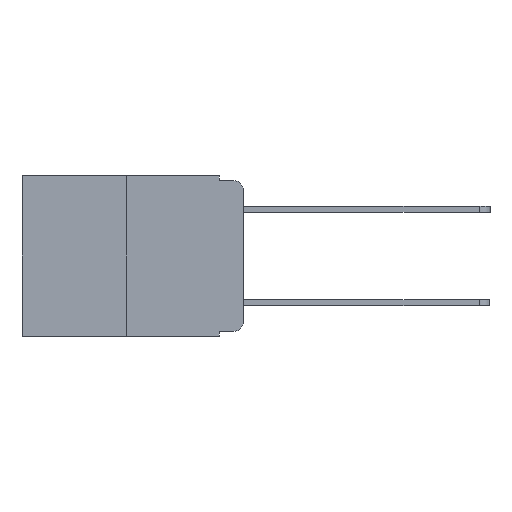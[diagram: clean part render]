
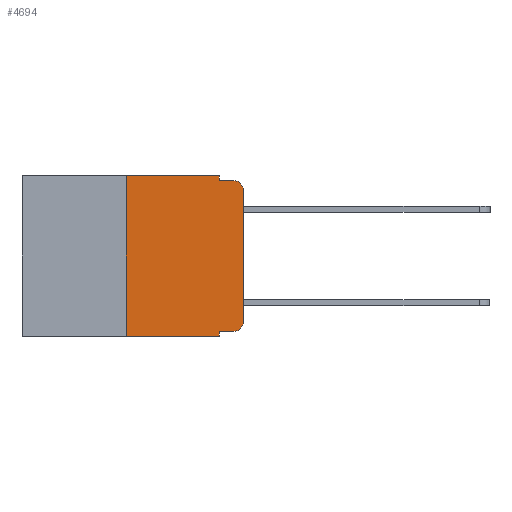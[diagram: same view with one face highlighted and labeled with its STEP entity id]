
A CAD part, left-side view. The second image highlights one B-rep face of the part: STEP entity #4694.
In plain terms, the highlighted planar face has unit normal (-1, 0, 0).
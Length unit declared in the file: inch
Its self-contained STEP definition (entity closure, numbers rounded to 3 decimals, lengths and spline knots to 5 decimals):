
#53 = VERTEX_POINT ( 'NONE', #17439 ) ;
#73 = LINE ( 'NONE', #3308, #14886 ) ;
#321 = VERTEX_POINT ( 'NONE', #8775 ) ;
#516 = VERTEX_POINT ( 'NONE', #12780 ) ;
#943 = CARTESIAN_POINT ( 'NONE',  ( 0., 0.02, -0.01 ) ) ;
#1079 = EDGE_CURVE ( 'NONE', #13276, #7350, #13973, .T. ) ;
#1760 = CARTESIAN_POINT ( 'NONE',  ( 0., 0.051, -0.333 ) ) ;
#1866 = VECTOR ( 'NONE', #15517, 39.37008 ) ;
#1923 = CARTESIAN_POINT ( 'NONE',  ( 0., 0.051, -0.01 ) ) ;
#2080 = EDGE_CURVE ( 'NONE', #9093, #53, #17337, .T. ) ;
#3308 = CARTESIAN_POINT ( 'NONE',  ( 0., 0.25, 0. ) ) ;
#3718 = VERTEX_POINT ( 'NONE', #943 ) ;
#3802 = VERTEX_POINT ( 'NONE', #11921 ) ;
#4694 = ADVANCED_FACE ( 'NONE', ( #8279 ), #8007, .F. ) ;
#4800 = EDGE_CURVE ( 'NONE', #3802, #321, #13124, .T. ) ;
#4819 = CARTESIAN_POINT ( 'NONE',  ( 0., 0.051, -0.333 ) ) ;
#4912 = VECTOR ( 'NONE', #18593, 39.37008 ) ;
#4969 = LINE ( 'NONE', #14575, #16102 ) ;
#5152 = EDGE_CURVE ( 'NONE', #516, #3718, #18924, .T. ) ;
#5221 = VECTOR ( 'NONE', #10815, 39.37008 ) ;
#5332 = ORIENTED_EDGE ( 'NONE', *, *, #12474, .T. ) ;
#5348 = DIRECTION ( 'NONE',  ( 0., -1., 0. ) ) ;
#6145 = EDGE_LOOP ( 'NONE', ( #15841, #15179, #15151, #14642, #14334, #14672, #7947, #7739, #6609, #5332 ) ) ;
#6278 = DIRECTION ( 'NONE',  ( -1., 0., 0. ) ) ;
#6318 = CARTESIAN_POINT ( 'NONE',  ( 0., 0.02, -0.333 ) ) ;
#6609 = ORIENTED_EDGE ( 'NONE', *, *, #16729, .T. ) ;
#6822 = CARTESIAN_POINT ( 'NONE',  ( 0., 0.02, -0.03 ) ) ;
#7215 = VERTEX_POINT ( 'NONE', #6318 ) ;
#7350 = VERTEX_POINT ( 'NONE', #9865 ) ;
#7522 = CIRCLE ( 'NONE', #13539, 0.02 ) ;
#7739 = ORIENTED_EDGE ( 'NONE', *, *, #16556, .F. ) ;
#7822 = LINE ( 'NONE', #1760, #18480 ) ;
#7947 = ORIENTED_EDGE ( 'NONE', *, *, #1079, .T. ) ;
#7963 = CARTESIAN_POINT ( 'NONE',  ( 0., 0.473, 0. ) ) ;
#8007 = PLANE ( 'NONE',  #8493 ) ;
#8279 = FACE_OUTER_BOUND ( 'NONE', #6145, .T. ) ;
#8397 = DIRECTION ( 'NONE',  ( 0., 0., -1. ) ) ;
#8493 = AXIS2_PLACEMENT_3D ( 'NONE', #7963, #9021, #8964 ) ;
#8775 = CARTESIAN_POINT ( 'NONE',  ( 0., 0.051, 0. ) ) ;
#8964 = DIRECTION ( 'NONE',  ( 0., 0., -1. ) ) ;
#9021 = DIRECTION ( 'NONE',  ( 1., 0., 0. ) ) ;
#9029 = EDGE_CURVE ( 'NONE', #13276, #3802, #73, .T. ) ;
#9093 = VERTEX_POINT ( 'NONE', #11124 ) ;
#9163 = EDGE_CURVE ( 'NONE', #53, #3718, #10747, .T. ) ;
#9364 = LINE ( 'NONE', #17678, #5221 ) ;
#9378 = VECTOR ( 'NONE', #5348, 39.37008 ) ;
#9865 = CARTESIAN_POINT ( 'NONE',  ( 0., 0.051, -0.343 ) ) ;
#10607 = DIRECTION ( 'NONE',  ( 0., -1., 0. ) ) ;
#10747 = CIRCLE ( 'NONE', #12234, 0.02 ) ;
#10815 = DIRECTION ( 'NONE',  ( 0., 0., -1. ) ) ;
#11124 = CARTESIAN_POINT ( 'NONE',  ( 0., 0., -0.313 ) ) ;
#11921 = CARTESIAN_POINT ( 'NONE',  ( 0., 0.25, 0. ) ) ;
#12234 = AXIS2_PLACEMENT_3D ( 'NONE', #6822, #16710, #8397 ) ;
#12474 = EDGE_CURVE ( 'NONE', #7215, #9093, #7522, .T. ) ;
#12527 = DIRECTION ( 'NONE',  ( 0., -1., 0. ) ) ;
#12780 = CARTESIAN_POINT ( 'NONE',  ( 0., 0.051, -0.01 ) ) ;
#13124 = LINE ( 'NONE', #17218, #9378 ) ;
#13211 = DIRECTION ( 'NONE',  ( 0., 0., -1. ) ) ;
#13276 = VERTEX_POINT ( 'NONE', #17198 ) ;
#13539 = AXIS2_PLACEMENT_3D ( 'NONE', #14904, #6278, #16261 ) ;
#13973 = LINE ( 'NONE', #15211, #1866 ) ;
#14334 = ORIENTED_EDGE ( 'NONE', *, *, #4800, .F. ) ;
#14575 = CARTESIAN_POINT ( 'NONE',  ( 0., 0.051, 0. ) ) ;
#14642 = ORIENTED_EDGE ( 'NONE', *, *, #16252, .F. ) ;
#14672 = ORIENTED_EDGE ( 'NONE', *, *, #9029, .F. ) ;
#14886 = VECTOR ( 'NONE', #17926, 39.37008 ) ;
#14904 = CARTESIAN_POINT ( 'NONE',  ( 0., 0.02, -0.313 ) ) ;
#15151 = ORIENTED_EDGE ( 'NONE', *, *, #5152, .F. ) ;
#15179 = ORIENTED_EDGE ( 'NONE', *, *, #9163, .T. ) ;
#15211 = CARTESIAN_POINT ( 'NONE',  ( 0., 0.473, -0.343 ) ) ;
#15284 = VECTOR ( 'NONE', #10607, 39.37008 ) ;
#15517 = DIRECTION ( 'NONE',  ( 0., -1., 0. ) ) ;
#15841 = ORIENTED_EDGE ( 'NONE', *, *, #2080, .T. ) ;
#16102 = VECTOR ( 'NONE', #13211, 39.37008 ) ;
#16252 = EDGE_CURVE ( 'NONE', #321, #516, #4969, .T. ) ;
#16261 = DIRECTION ( 'NONE',  ( 0., 0., -1. ) ) ;
#16412 = CARTESIAN_POINT ( 'NONE',  ( 0., 0., 0. ) ) ;
#16556 = EDGE_CURVE ( 'NONE', #18759, #7350, #9364, .T. ) ;
#16710 = DIRECTION ( 'NONE',  ( -1., 0., 0. ) ) ;
#16729 = EDGE_CURVE ( 'NONE', #18759, #7215, #7822, .T. ) ;
#17198 = CARTESIAN_POINT ( 'NONE',  ( 0., 0.25, -0.343 ) ) ;
#17218 = CARTESIAN_POINT ( 'NONE',  ( 0., 0.473, 0. ) ) ;
#17337 = LINE ( 'NONE', #16412, #4912 ) ;
#17439 = CARTESIAN_POINT ( 'NONE',  ( 0., 0., -0.03 ) ) ;
#17678 = CARTESIAN_POINT ( 'NONE',  ( 0., 0.051, 0. ) ) ;
#17926 = DIRECTION ( 'NONE',  ( 0., 0., 1. ) ) ;
#18480 = VECTOR ( 'NONE', #12527, 39.37008 ) ;
#18593 = DIRECTION ( 'NONE',  ( 0., 0., 1. ) ) ;
#18759 = VERTEX_POINT ( 'NONE', #4819 ) ;
#18924 = LINE ( 'NONE', #1923, #15284 ) ;
